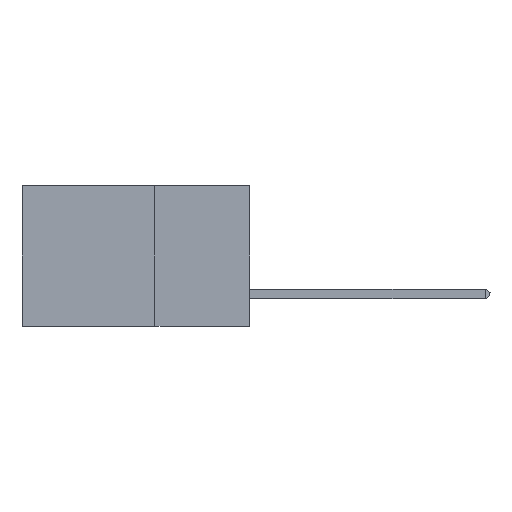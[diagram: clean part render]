
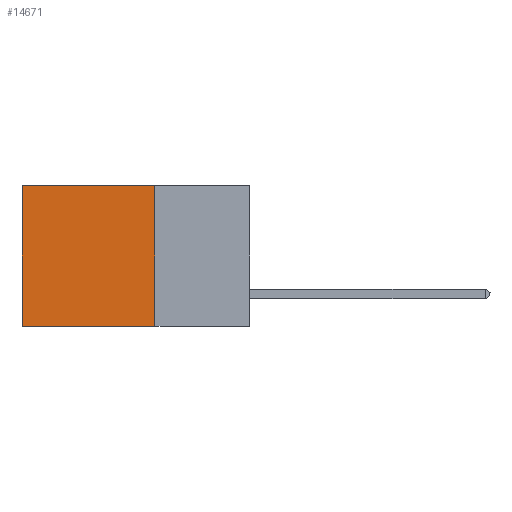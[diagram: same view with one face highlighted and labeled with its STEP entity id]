
A CAD part, left-side view. The second image highlights one B-rep face of the part: STEP entity #14671.
In plain terms, the highlighted planar face has unit normal (-1, 0, 0).
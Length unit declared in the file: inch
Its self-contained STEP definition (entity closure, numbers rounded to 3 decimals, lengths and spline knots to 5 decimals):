
#560 = CARTESIAN_POINT ( 'NONE',  ( 0.2875, 0.6, 0. ) ) ;
#595 = DIRECTION ( 'NONE',  ( 0., 0., -1. ) ) ;
#5335 = LINE ( 'NONE', #560, #12745 ) ;
#6096 = CARTESIAN_POINT ( 'NONE',  ( 0.2875, 0.6, 0. ) ) ;
#6481 = DIRECTION ( 'NONE',  ( 0., 0., -1. ) ) ;
#6507 = DIRECTION ( 'NONE',  ( 0., 1., 0. ) ) ;
#7411 = ORIENTED_EDGE ( 'NONE', *, *, #16938, .T. ) ;
#8063 = EDGE_CURVE ( 'NONE', #22759, #15722, #10845, .T. ) ;
#8066 = ORIENTED_EDGE ( 'NONE', *, *, #16557, .T. ) ;
#8693 = CARTESIAN_POINT ( 'NONE',  ( 0.2875, 0.25, 0. ) ) ;
#8864 = EDGE_LOOP ( 'NONE', ( #8066, #20484, #18732, #7411 ) ) ;
#9227 = DIRECTION ( 'NONE',  ( 0., 1., 0. ) ) ;
#9423 = VECTOR ( 'NONE', #9227, 39.37008 ) ;
#9797 = CARTESIAN_POINT ( 'NONE',  ( 0.2875, 0.6, -0.37 ) ) ;
#9833 = DIRECTION ( 'NONE',  ( 1., 0., 0. ) ) ;
#10324 = VERTEX_POINT ( 'NONE', #17702 ) ;
#10845 = LINE ( 'NONE', #16432, #9423 ) ;
#11743 = FACE_OUTER_BOUND ( 'NONE', #8864, .T. ) ;
#11815 = LINE ( 'NONE', #8693, #22945 ) ;
#12723 = LINE ( 'NONE', #13861, #14437 ) ;
#12745 = VECTOR ( 'NONE', #6481, 39.37008 ) ;
#13237 = PLANE ( 'NONE',  #14147 ) ;
#13287 = EDGE_CURVE ( 'NONE', #10324, #22759, #11815, .T. ) ;
#13861 = CARTESIAN_POINT ( 'NONE',  ( 0.2875, 0.25, 0. ) ) ;
#14147 = AXIS2_PLACEMENT_3D ( 'NONE', #15143, #9833, #595 ) ;
#14437 = VECTOR ( 'NONE', #6507, 39.37008 ) ;
#14671 = ADVANCED_FACE ( 'NONE', ( #11743 ), #13237, .F. ) ;
#15143 = CARTESIAN_POINT ( 'NONE',  ( 0.2875, 0.25, 0. ) ) ;
#15722 = VERTEX_POINT ( 'NONE', #9797 ) ;
#16432 = CARTESIAN_POINT ( 'NONE',  ( 0.2875, 0.25, -0.37 ) ) ;
#16557 = EDGE_CURVE ( 'NONE', #19259, #15722, #5335, .T. ) ;
#16938 = EDGE_CURVE ( 'NONE', #10324, #19259, #12723, .T. ) ;
#17702 = CARTESIAN_POINT ( 'NONE',  ( 0.2875, 0.25, 0. ) ) ;
#17795 = DIRECTION ( 'NONE',  ( 0., 0., -1. ) ) ;
#18732 = ORIENTED_EDGE ( 'NONE', *, *, #13287, .F. ) ;
#19259 = VERTEX_POINT ( 'NONE', #6096 ) ;
#20484 = ORIENTED_EDGE ( 'NONE', *, *, #8063, .F. ) ;
#22444 = CARTESIAN_POINT ( 'NONE',  ( 0.2875, 0.25, -0.37 ) ) ;
#22759 = VERTEX_POINT ( 'NONE', #22444 ) ;
#22945 = VECTOR ( 'NONE', #17795, 39.37008 ) ;
